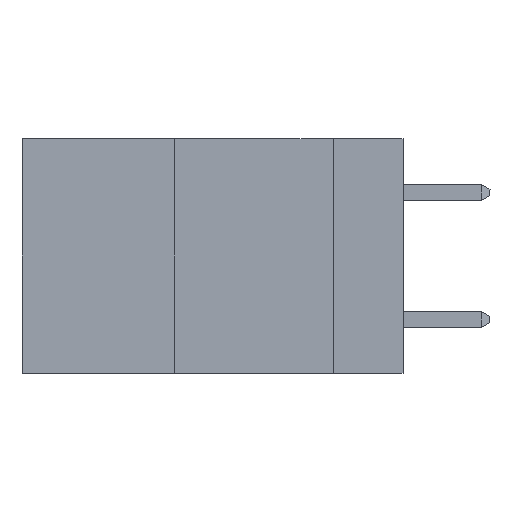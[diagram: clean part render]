
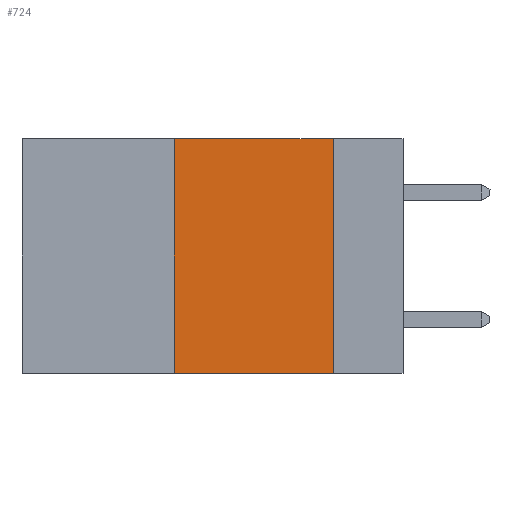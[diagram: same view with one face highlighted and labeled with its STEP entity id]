
A CAD part, left-side view. The second image highlights one B-rep face of the part: STEP entity #724.
In plain terms, the highlighted planar face has unit normal (-1, 0, 0).
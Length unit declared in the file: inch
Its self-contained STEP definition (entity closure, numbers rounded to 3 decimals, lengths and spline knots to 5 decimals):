
#215 = ORIENTED_EDGE ( 'NONE', *, *, #2005, .F. ) ;
#550 = VECTOR ( 'NONE', #1146, 39.37008 ) ;
#724 = ADVANCED_FACE ( 'NONE', ( #9625 ), #13050, .F. ) ;
#1146 = DIRECTION ( 'NONE',  ( 0., 0., 1. ) ) ;
#1386 = VERTEX_POINT ( 'NONE', #2329 ) ;
#1406 = EDGE_LOOP ( 'NONE', ( #4400, #215, #11783, #2425 ) ) ;
#1815 = VERTEX_POINT ( 'NONE', #4100 ) ;
#2005 = EDGE_CURVE ( 'NONE', #6294, #8510, #10300, .T. ) ;
#2329 = CARTESIAN_POINT ( 'NONE',  ( 0., 0.11, -0.37 ) ) ;
#2425 = ORIENTED_EDGE ( 'NONE', *, *, #8181, .T. ) ;
#2667 = CARTESIAN_POINT ( 'NONE',  ( 0., 0.6, -0.37 ) ) ;
#2813 = CARTESIAN_POINT ( 'NONE',  ( 0., 0.6, 0. ) ) ;
#3177 = VECTOR ( 'NONE', #14238, 39.37008 ) ;
#3484 = DIRECTION ( 'NONE',  ( 0., -1., 0. ) ) ;
#4100 = CARTESIAN_POINT ( 'NONE',  ( 0., 0.36, -0.37 ) ) ;
#4358 = LINE ( 'NONE', #5475, #550 ) ;
#4400 = ORIENTED_EDGE ( 'NONE', *, *, #12137, .F. ) ;
#5233 = LINE ( 'NONE', #2667, #3177 ) ;
#5249 = CARTESIAN_POINT ( 'NONE',  ( 0., 0.36, 0. ) ) ;
#5475 = CARTESIAN_POINT ( 'NONE',  ( 0., 0.36, 0. ) ) ;
#6294 = VERTEX_POINT ( 'NONE', #5249 ) ;
#6323 = CARTESIAN_POINT ( 'NONE',  ( 0., 0.11, 0. ) ) ;
#6965 = DIRECTION ( 'NONE',  ( 0., 0., -1. ) ) ;
#7814 = VECTOR ( 'NONE', #3484, 39.37008 ) ;
#8181 = EDGE_CURVE ( 'NONE', #1815, #1386, #5233, .T. ) ;
#8510 = VERTEX_POINT ( 'NONE', #6323 ) ;
#8642 = CARTESIAN_POINT ( 'NONE',  ( 0., 0.6, 0. ) ) ;
#9625 = FACE_OUTER_BOUND ( 'NONE', #1406, .T. ) ;
#9675 = EDGE_CURVE ( 'NONE', #1815, #6294, #4358, .T. ) ;
#10077 = VECTOR ( 'NONE', #6965, 39.37008 ) ;
#10300 = LINE ( 'NONE', #2813, #7814 ) ;
#10904 = DIRECTION ( 'NONE',  ( 1., 0., 0. ) ) ;
#11783 = ORIENTED_EDGE ( 'NONE', *, *, #9675, .F. ) ;
#12137 = EDGE_CURVE ( 'NONE', #8510, #1386, #13742, .T. ) ;
#12205 = AXIS2_PLACEMENT_3D ( 'NONE', #8642, #10904, #13329 ) ;
#12632 = CARTESIAN_POINT ( 'NONE',  ( 0., 0.11, 0. ) ) ;
#13050 = PLANE ( 'NONE',  #12205 ) ;
#13329 = DIRECTION ( 'NONE',  ( 0., 0., -1. ) ) ;
#13742 = LINE ( 'NONE', #12632, #10077 ) ;
#14238 = DIRECTION ( 'NONE',  ( 0., -1., 0. ) ) ;
